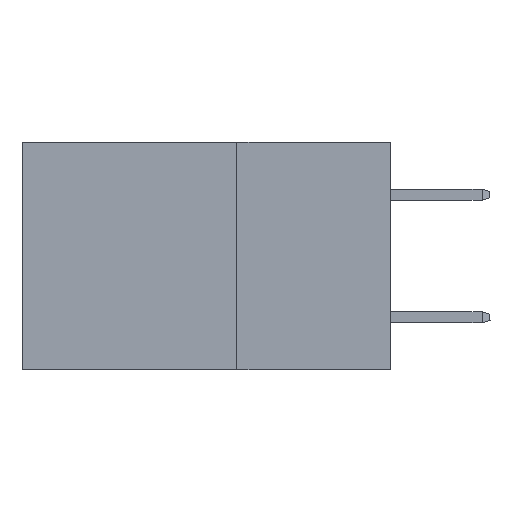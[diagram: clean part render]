
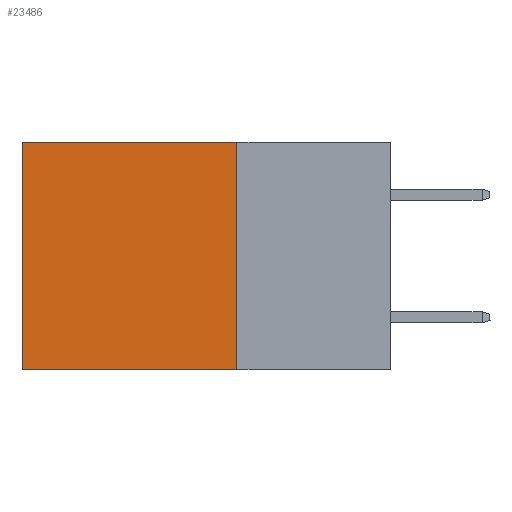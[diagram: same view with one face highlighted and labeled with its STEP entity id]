
A CAD part, left-side view. The second image highlights one B-rep face of the part: STEP entity #23486.
In plain terms, the highlighted planar face has unit normal (-1, 0, 0).
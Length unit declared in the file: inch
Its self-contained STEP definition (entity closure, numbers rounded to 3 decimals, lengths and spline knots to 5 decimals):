
#179 = LINE ( 'NONE', #7184, #11919 ) ;
#644 = CARTESIAN_POINT ( 'NONE',  ( 0.2875, 0.6, 0. ) ) ;
#897 = VERTEX_POINT ( 'NONE', #11651 ) ;
#2357 = DIRECTION ( 'NONE',  ( 0., 1., 0. ) ) ;
#3350 = VERTEX_POINT ( 'NONE', #24922 ) ;
#5032 = VERTEX_POINT ( 'NONE', #14239 ) ;
#5500 = LINE ( 'NONE', #17549, #29031 ) ;
#6293 = DIRECTION ( 'NONE',  ( 0., 1., 0. ) ) ;
#6697 = EDGE_LOOP ( 'NONE', ( #23459, #9992, #25748, #26824 ) ) ;
#6820 = LINE ( 'NONE', #644, #20130 ) ;
#7184 = CARTESIAN_POINT ( 'NONE',  ( 0.2875, 0.25, 0. ) ) ;
#7880 = PLANE ( 'NONE',  #7881 ) ;
#7881 = AXIS2_PLACEMENT_3D ( 'NONE', #30873, #25424, #13097 ) ;
#7941 = LINE ( 'NONE', #19210, #26415 ) ;
#9992 = ORIENTED_EDGE ( 'NONE', *, *, #13166, .F. ) ;
#10530 = VERTEX_POINT ( 'NONE', #30822 ) ;
#11651 = CARTESIAN_POINT ( 'NONE',  ( 0.2875, 0.25, -0.37 ) ) ;
#11919 = VECTOR ( 'NONE', #24943, 39.37008 ) ;
#12987 = DIRECTION ( 'NONE',  ( 0., 0., -1. ) ) ;
#13097 = DIRECTION ( 'NONE',  ( 0., 0., -1. ) ) ;
#13166 = EDGE_CURVE ( 'NONE', #897, #5032, #5500, .T. ) ;
#14037 = FACE_OUTER_BOUND ( 'NONE', #6697, .T. ) ;
#14239 = CARTESIAN_POINT ( 'NONE',  ( 0.2875, 0.6, -0.37 ) ) ;
#17549 = CARTESIAN_POINT ( 'NONE',  ( 0.2875, 0.25, -0.37 ) ) ;
#19210 = CARTESIAN_POINT ( 'NONE',  ( 0.2875, 0.25, 0. ) ) ;
#20130 = VECTOR ( 'NONE', #12987, 39.37008 ) ;
#22623 = EDGE_CURVE ( 'NONE', #10530, #897, #179, .T. ) ;
#23459 = ORIENTED_EDGE ( 'NONE', *, *, #29710, .T. ) ;
#23486 = ADVANCED_FACE ( 'NONE', ( #14037 ), #7880, .F. ) ;
#24922 = CARTESIAN_POINT ( 'NONE',  ( 0.2875, 0.6, 0. ) ) ;
#24943 = DIRECTION ( 'NONE',  ( 0., 0., -1. ) ) ;
#25424 = DIRECTION ( 'NONE',  ( 1., 0., 0. ) ) ;
#25748 = ORIENTED_EDGE ( 'NONE', *, *, #22623, .F. ) ;
#26415 = VECTOR ( 'NONE', #6293, 39.37008 ) ;
#26824 = ORIENTED_EDGE ( 'NONE', *, *, #27660, .T. ) ;
#27660 = EDGE_CURVE ( 'NONE', #10530, #3350, #7941, .T. ) ;
#29031 = VECTOR ( 'NONE', #2357, 39.37008 ) ;
#29710 = EDGE_CURVE ( 'NONE', #3350, #5032, #6820, .T. ) ;
#30822 = CARTESIAN_POINT ( 'NONE',  ( 0.2875, 0.25, 0. ) ) ;
#30873 = CARTESIAN_POINT ( 'NONE',  ( 0.2875, 0.25, 0. ) ) ;
